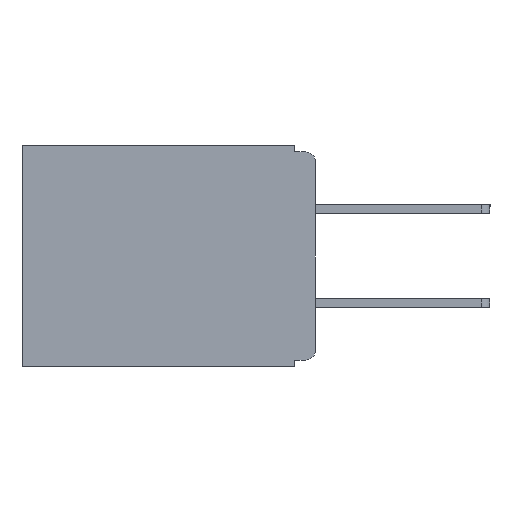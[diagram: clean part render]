
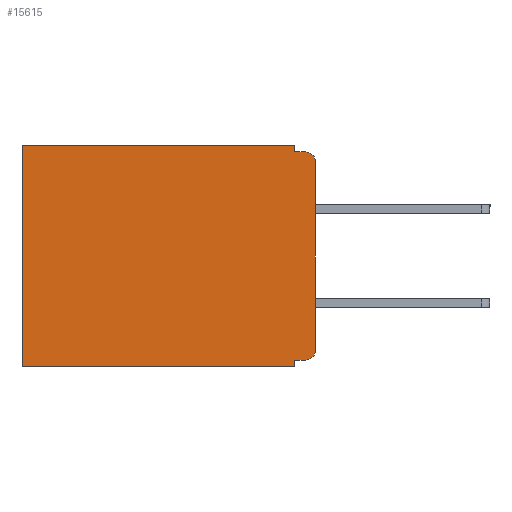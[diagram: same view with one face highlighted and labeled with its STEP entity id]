
A CAD part, left-side view. The second image highlights one B-rep face of the part: STEP entity #15615.
In plain terms, the highlighted planar face has unit normal (-1, 0, 0).
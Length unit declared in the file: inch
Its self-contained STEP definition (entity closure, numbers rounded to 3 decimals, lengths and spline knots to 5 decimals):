
#222 = LINE ( 'NONE', #6416, #17483 ) ;
#285 = LINE ( 'NONE', #19487, #13299 ) ;
#857 = EDGE_CURVE ( 'NONE', #1714, #12971, #5969, .T. ) ;
#936 = DIRECTION ( 'NONE',  ( 0., 1., 0. ) ) ;
#995 = CARTESIAN_POINT ( 'NONE',  ( 0.3, 0.031, 0. ) ) ;
#1243 = PLANE ( 'NONE',  #8086 ) ;
#1298 = CARTESIAN_POINT ( 'NONE',  ( 0.3, 0., -0.32 ) ) ;
#1424 = ORIENTED_EDGE ( 'NONE', *, *, #18648, .F. ) ;
#1481 = DIRECTION ( 'NONE',  ( 0., -1., 0. ) ) ;
#1714 = VERTEX_POINT ( 'NONE', #8082 ) ;
#1938 = CARTESIAN_POINT ( 'NONE',  ( 0.3, 0.015, -0.32 ) ) ;
#1951 = VERTEX_POINT ( 'NONE', #8290 ) ;
#2271 = CARTESIAN_POINT ( 'NONE',  ( 0.3, 0., -0.025 ) ) ;
#2618 = LINE ( 'NONE', #995, #11173 ) ;
#4205 = EDGE_CURVE ( 'NONE', #12971, #7862, #285, .T. ) ;
#4540 = DIRECTION ( 'NONE',  ( 1., 0., 0. ) ) ;
#4886 = CARTESIAN_POINT ( 'NONE',  ( 0.3, 0., -0.305 ) ) ;
#5969 = LINE ( 'NONE', #20313, #10078 ) ;
#5978 = CIRCLE ( 'NONE', #13401, 0.015 ) ;
#6107 = ORIENTED_EDGE ( 'NONE', *, *, #9476, .T. ) ;
#6416 = CARTESIAN_POINT ( 'NONE',  ( 0.3, 0., -0.01 ) ) ;
#7862 = VERTEX_POINT ( 'NONE', #13139 ) ;
#7863 = VECTOR ( 'NONE', #21201, 39.37008 ) ;
#7953 = DIRECTION ( 'NONE',  ( -1., 0., 0. ) ) ;
#8082 = CARTESIAN_POINT ( 'NONE',  ( 0.3, 0.031, -0.32 ) ) ;
#8086 = AXIS2_PLACEMENT_3D ( 'NONE', #14788, #4540, #16395 ) ;
#8290 = CARTESIAN_POINT ( 'NONE',  ( 0.3, 0.437, 0. ) ) ;
#8532 = CARTESIAN_POINT ( 'NONE',  ( 0.3, 0.015, -0.01 ) ) ;
#8754 = ORIENTED_EDGE ( 'NONE', *, *, #11399, .T. ) ;
#9476 = EDGE_CURVE ( 'NONE', #18763, #1951, #13410, .T. ) ;
#9614 = CARTESIAN_POINT ( 'NONE',  ( 0.3, 0.015, -0.025 ) ) ;
#9829 = ORIENTED_EDGE ( 'NONE', *, *, #17990, .T. ) ;
#10078 = VECTOR ( 'NONE', #15830, 39.37008 ) ;
#10505 = ORIENTED_EDGE ( 'NONE', *, *, #12001, .F. ) ;
#10615 = LINE ( 'NONE', #1298, #14555 ) ;
#10873 = LINE ( 'NONE', #17789, #19035 ) ;
#10895 = VERTEX_POINT ( 'NONE', #16656 ) ;
#11173 = VECTOR ( 'NONE', #12877, 39.37008 ) ;
#11326 = EDGE_CURVE ( 'NONE', #18763, #10895, #2618, .T. ) ;
#11340 = DIRECTION ( 'NONE',  ( 0., 0., -1. ) ) ;
#11399 = EDGE_CURVE ( 'NONE', #21295, #18760, #5978, .T. ) ;
#11758 = VERTEX_POINT ( 'NONE', #8532 ) ;
#12001 = EDGE_CURVE ( 'NONE', #16623, #18760, #10873, .T. ) ;
#12087 = ORIENTED_EDGE ( 'NONE', *, *, #4205, .F. ) ;
#12877 = DIRECTION ( 'NONE',  ( 0., 0., -1. ) ) ;
#12882 = ORIENTED_EDGE ( 'NONE', *, *, #11326, .F. ) ;
#12971 = VERTEX_POINT ( 'NONE', #13681 ) ;
#13088 = AXIS2_PLACEMENT_3D ( 'NONE', #9614, #21071, #11340 ) ;
#13139 = CARTESIAN_POINT ( 'NONE',  ( 0.3, 0.437, -0.33 ) ) ;
#13215 = DIRECTION ( 'NONE',  ( 0., 1., 0. ) ) ;
#13299 = VECTOR ( 'NONE', #936, 39.37008 ) ;
#13401 = AXIS2_PLACEMENT_3D ( 'NONE', #17945, #7953, #19540 ) ;
#13410 = LINE ( 'NONE', #16201, #16675 ) ;
#13681 = CARTESIAN_POINT ( 'NONE',  ( 0.3, 0.031, -0.33 ) ) ;
#14555 = VECTOR ( 'NONE', #13215, 39.37008 ) ;
#14788 = CARTESIAN_POINT ( 'NONE',  ( 0.3, 0., -0.33 ) ) ;
#14841 = CIRCLE ( 'NONE', #13088, 0.015 ) ;
#15048 = EDGE_CURVE ( 'NONE', #10895, #11758, #222, .T. ) ;
#15456 = FACE_OUTER_BOUND ( 'NONE', #20000, .T. ) ;
#15615 = ADVANCED_FACE ( 'NONE', ( #15456 ), #1243, .F. ) ;
#15830 = DIRECTION ( 'NONE',  ( 0., 0., -1. ) ) ;
#16201 = CARTESIAN_POINT ( 'NONE',  ( 0.3, 0., 0. ) ) ;
#16395 = DIRECTION ( 'NONE',  ( 0., 0., -1. ) ) ;
#16473 = CARTESIAN_POINT ( 'NONE',  ( 0.3, 0.437, -0.33 ) ) ;
#16623 = VERTEX_POINT ( 'NONE', #2271 ) ;
#16656 = CARTESIAN_POINT ( 'NONE',  ( 0.3, 0.031, -0.01 ) ) ;
#16675 = VECTOR ( 'NONE', #19387, 39.37008 ) ;
#17319 = LINE ( 'NONE', #16473, #7863 ) ;
#17483 = VECTOR ( 'NONE', #1481, 39.37008 ) ;
#17789 = CARTESIAN_POINT ( 'NONE',  ( 0.3, 0., -0.33 ) ) ;
#17945 = CARTESIAN_POINT ( 'NONE',  ( 0.3, 0.015, -0.305 ) ) ;
#17990 = EDGE_CURVE ( 'NONE', #16623, #11758, #14841, .T. ) ;
#18648 = EDGE_CURVE ( 'NONE', #21295, #1714, #10615, .T. ) ;
#18760 = VERTEX_POINT ( 'NONE', #4886 ) ;
#18763 = VERTEX_POINT ( 'NONE', #19913 ) ;
#19035 = VECTOR ( 'NONE', #19368, 39.37008 ) ;
#19260 = ORIENTED_EDGE ( 'NONE', *, *, #857, .F. ) ;
#19368 = DIRECTION ( 'NONE',  ( 0., 0., -1. ) ) ;
#19387 = DIRECTION ( 'NONE',  ( 0., 1., 0. ) ) ;
#19453 = ORIENTED_EDGE ( 'NONE', *, *, #20572, .T. ) ;
#19487 = CARTESIAN_POINT ( 'NONE',  ( 0.3, 0., -0.33 ) ) ;
#19540 = DIRECTION ( 'NONE',  ( 0., 0., -1. ) ) ;
#19913 = CARTESIAN_POINT ( 'NONE',  ( 0.3, 0.031, 0. ) ) ;
#20000 = EDGE_LOOP ( 'NONE', ( #10505, #9829, #20285, #12882, #6107, #19453, #12087, #19260, #1424, #8754 ) ) ;
#20285 = ORIENTED_EDGE ( 'NONE', *, *, #15048, .F. ) ;
#20313 = CARTESIAN_POINT ( 'NONE',  ( 0.3, 0.031, -0.33 ) ) ;
#20572 = EDGE_CURVE ( 'NONE', #1951, #7862, #17319, .T. ) ;
#21071 = DIRECTION ( 'NONE',  ( -1., 0., 0. ) ) ;
#21201 = DIRECTION ( 'NONE',  ( 0., 0., -1. ) ) ;
#21295 = VERTEX_POINT ( 'NONE', #1938 ) ;
